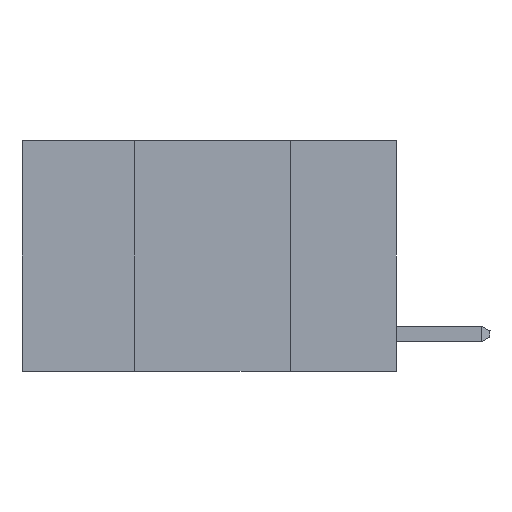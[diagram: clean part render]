
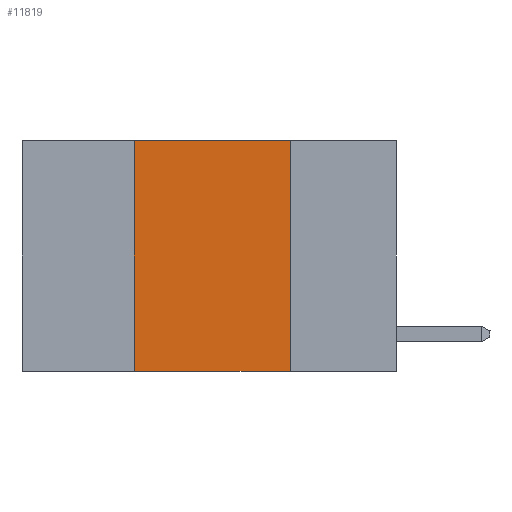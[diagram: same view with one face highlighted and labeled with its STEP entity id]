
A CAD part, left-side view. The second image highlights one B-rep face of the part: STEP entity #11819.
In plain terms, the highlighted planar face has unit normal (-1, 0, 0).
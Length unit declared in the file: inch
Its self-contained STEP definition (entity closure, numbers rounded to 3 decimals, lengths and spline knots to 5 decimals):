
#585 = LINE ( 'NONE', #23246, #20225 ) ;
#641 = VERTEX_POINT ( 'NONE', #21562 ) ;
#1195 = EDGE_LOOP ( 'NONE', ( #20935, #12779, #15283, #19864 ) ) ;
#3092 = CARTESIAN_POINT ( 'NONE',  ( 0., 0.6, -0.37 ) ) ;
#3110 = VERTEX_POINT ( 'NONE', #10325 ) ;
#3600 = VECTOR ( 'NONE', #12955, 39.37008 ) ;
#5011 = DIRECTION ( 'NONE',  ( 0., 0., -1. ) ) ;
#5127 = PLANE ( 'NONE',  #18775 ) ;
#6324 = VERTEX_POINT ( 'NONE', #8421 ) ;
#8095 = EDGE_CURVE ( 'NONE', #6324, #3110, #19959, .T. ) ;
#8413 = LINE ( 'NONE', #29834, #14469 ) ;
#8421 = CARTESIAN_POINT ( 'NONE',  ( 0., 0.42, -0.37 ) ) ;
#9214 = DIRECTION ( 'NONE',  ( 0., 0., -1. ) ) ;
#10325 = CARTESIAN_POINT ( 'NONE',  ( 0., 0.42, 0. ) ) ;
#11399 = EDGE_CURVE ( 'NONE', #26703, #641, #585, .T. ) ;
#11819 = ADVANCED_FACE ( 'NONE', ( #27772 ), #5127, .F. ) ;
#12385 = DIRECTION ( 'NONE',  ( 0., -1., 0. ) ) ;
#12779 = ORIENTED_EDGE ( 'NONE', *, *, #13783, .F. ) ;
#12955 = DIRECTION ( 'NONE',  ( 0., 0., 1. ) ) ;
#13106 = CARTESIAN_POINT ( 'NONE',  ( 0., 0.42, 0. ) ) ;
#13735 = EDGE_CURVE ( 'NONE', #6324, #641, #23930, .T. ) ;
#13783 = EDGE_CURVE ( 'NONE', #3110, #26703, #8413, .T. ) ;
#14469 = VECTOR ( 'NONE', #29236, 39.37008 ) ;
#14531 = CARTESIAN_POINT ( 'NONE',  ( 0., 0.6, 0. ) ) ;
#15283 = ORIENTED_EDGE ( 'NONE', *, *, #8095, .F. ) ;
#17378 = VECTOR ( 'NONE', #12385, 39.37008 ) ;
#17755 = CARTESIAN_POINT ( 'NONE',  ( 0., 0.17, 0. ) ) ;
#18775 = AXIS2_PLACEMENT_3D ( 'NONE', #14531, #27927, #9214 ) ;
#19864 = ORIENTED_EDGE ( 'NONE', *, *, #13735, .T. ) ;
#19959 = LINE ( 'NONE', #13106, #3600 ) ;
#20225 = VECTOR ( 'NONE', #5011, 39.37008 ) ;
#20935 = ORIENTED_EDGE ( 'NONE', *, *, #11399, .F. ) ;
#21562 = CARTESIAN_POINT ( 'NONE',  ( 0., 0.17, -0.37 ) ) ;
#23246 = CARTESIAN_POINT ( 'NONE',  ( 0., 0.17, 0. ) ) ;
#23930 = LINE ( 'NONE', #3092, #17378 ) ;
#26703 = VERTEX_POINT ( 'NONE', #17755 ) ;
#27772 = FACE_OUTER_BOUND ( 'NONE', #1195, .T. ) ;
#27927 = DIRECTION ( 'NONE',  ( 1., 0., 0. ) ) ;
#29236 = DIRECTION ( 'NONE',  ( 0., -1., 0. ) ) ;
#29834 = CARTESIAN_POINT ( 'NONE',  ( 0., 0.6, 0. ) ) ;
